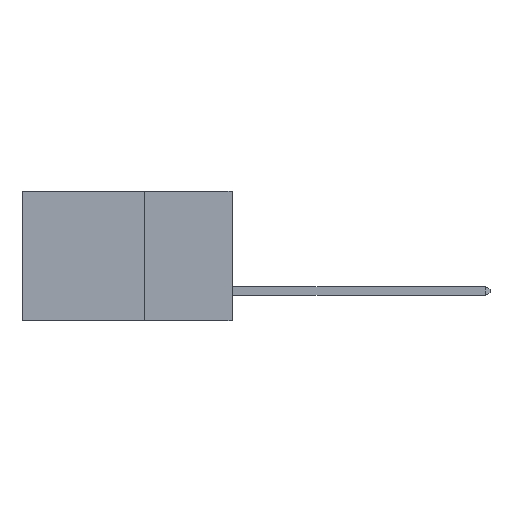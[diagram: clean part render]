
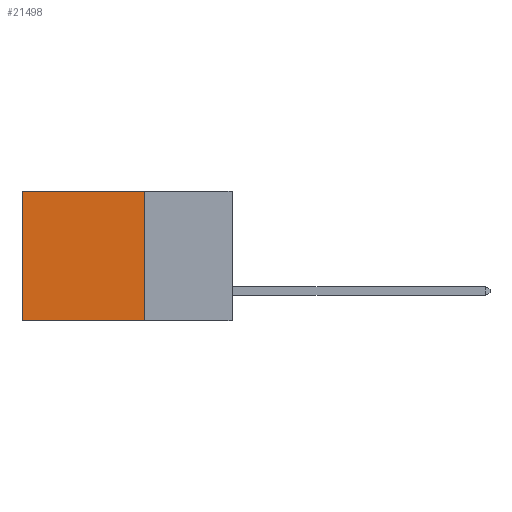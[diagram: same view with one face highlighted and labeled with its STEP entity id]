
A CAD part, left-side view. The second image highlights one B-rep face of the part: STEP entity #21498.
In plain terms, the highlighted planar face has unit normal (-1, 0, 0).
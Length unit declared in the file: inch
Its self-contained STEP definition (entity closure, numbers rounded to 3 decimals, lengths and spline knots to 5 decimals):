
#235 = DIRECTION ( 'NONE',  ( 0., 0., -1. ) ) ;
#1698 = VECTOR ( 'NONE', #6021, 39.37008 ) ;
#1902 = CARTESIAN_POINT ( 'NONE',  ( 0.2875, 0.25, 0. ) ) ;
#2051 = CARTESIAN_POINT ( 'NONE',  ( 0.2875, 0.25, 0. ) ) ;
#2310 = VECTOR ( 'NONE', #18353, 39.37008 ) ;
#3119 = CARTESIAN_POINT ( 'NONE',  ( 0.2875, 0.6, 0. ) ) ;
#3687 = EDGE_CURVE ( 'NONE', #8522, #16319, #17032, .T. ) ;
#3964 = VECTOR ( 'NONE', #21540, 39.37008 ) ;
#5259 = VERTEX_POINT ( 'NONE', #19548 ) ;
#5470 = LINE ( 'NONE', #18582, #2310 ) ;
#5599 = AXIS2_PLACEMENT_3D ( 'NONE', #1902, #6935, #235 ) ;
#6021 = DIRECTION ( 'NONE',  ( 0., 1., 0. ) ) ;
#6745 = DIRECTION ( 'NONE',  ( 0., 0., -1. ) ) ;
#6761 = FACE_OUTER_BOUND ( 'NONE', #21098, .T. ) ;
#6836 = VERTEX_POINT ( 'NONE', #2051 ) ;
#6935 = DIRECTION ( 'NONE',  ( 1., 0., 0. ) ) ;
#7781 = ORIENTED_EDGE ( 'NONE', *, *, #17101, .T. ) ;
#7888 = CARTESIAN_POINT ( 'NONE',  ( 0.2875, 0.6, 0. ) ) ;
#8522 = VERTEX_POINT ( 'NONE', #7888 ) ;
#9421 = ORIENTED_EDGE ( 'NONE', *, *, #3687, .T. ) ;
#10848 = LINE ( 'NONE', #11143, #1698 ) ;
#11143 = CARTESIAN_POINT ( 'NONE',  ( 0.2875, 0.25, -0.37 ) ) ;
#11503 = CARTESIAN_POINT ( 'NONE',  ( 0.2875, 0.6, -0.37 ) ) ;
#12869 = LINE ( 'NONE', #13477, #21484 ) ;
#13477 = CARTESIAN_POINT ( 'NONE',  ( 0.2875, 0.25, 0. ) ) ;
#16306 = ORIENTED_EDGE ( 'NONE', *, *, #17959, .F. ) ;
#16319 = VERTEX_POINT ( 'NONE', #11503 ) ;
#16890 = PLANE ( 'NONE',  #5599 ) ;
#17032 = LINE ( 'NONE', #3119, #3964 ) ;
#17101 = EDGE_CURVE ( 'NONE', #6836, #8522, #5470, .T. ) ;
#17959 = EDGE_CURVE ( 'NONE', #5259, #16319, #10848, .T. ) ;
#18353 = DIRECTION ( 'NONE',  ( 0., 1., 0. ) ) ;
#18376 = ORIENTED_EDGE ( 'NONE', *, *, #19862, .F. ) ;
#18582 = CARTESIAN_POINT ( 'NONE',  ( 0.2875, 0.25, 0. ) ) ;
#19548 = CARTESIAN_POINT ( 'NONE',  ( 0.2875, 0.25, -0.37 ) ) ;
#19862 = EDGE_CURVE ( 'NONE', #6836, #5259, #12869, .T. ) ;
#21098 = EDGE_LOOP ( 'NONE', ( #9421, #16306, #18376, #7781 ) ) ;
#21484 = VECTOR ( 'NONE', #6745, 39.37008 ) ;
#21498 = ADVANCED_FACE ( 'NONE', ( #6761 ), #16890, .F. ) ;
#21540 = DIRECTION ( 'NONE',  ( 0., 0., -1. ) ) ;
